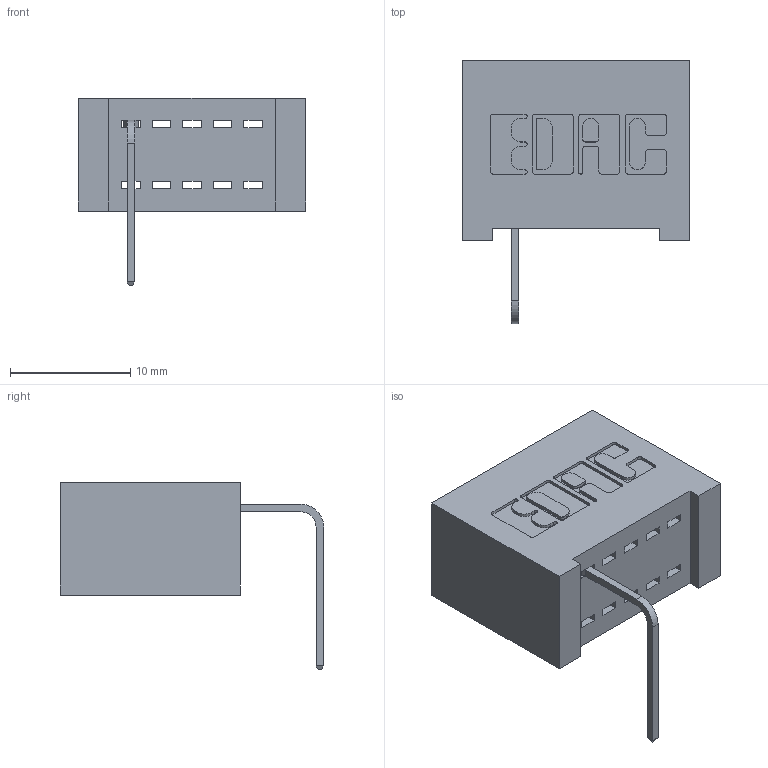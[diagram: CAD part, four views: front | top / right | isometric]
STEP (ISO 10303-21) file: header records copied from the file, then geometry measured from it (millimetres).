
FILE_DESCRIPTION (( 'STEP AP203' ), '1' );
FILE_NAME ('342-005-558-101.STEP', '2018-08-10T11:11:48', ( '' ), ( '' ), 'SwSTEP 2.0', 'SolidWorks 2016', '' );
FILE_SCHEMA (( 'CONFIG_CONTROL_DESIGN' ));
Length unit declared in the file: inch
Products named in the file (3): 342 Part_Lugless; 345-292-001_558 Tail - 2; 342-005-558-101
Assembly tree (2 placements, depth 2):
  342-005-558-101
    342 Part_Lugless
    345-292-001_558 Tail - 2
Bounding box: 18.95 x 21.91 x 15.62 mm (x, y, z)
Volume: 1891.7 mm3; surface area: 2192.2 mm2
Topology: 2 solids, 2 shells, 210 faces, 625 edges, 414 vertices
Faces by surface type: plane 154, cylinder 56
Entity records: 7389 total; most frequent: CARTESIAN_POINT 1305, ORIENTED_EDGE 1250, DIRECTION 1163, EDGE_CURVE 625, VECTOR 505, LINE 505, VERTEX_POINT 414, AXIS2_PLACEMENT_3D 329
